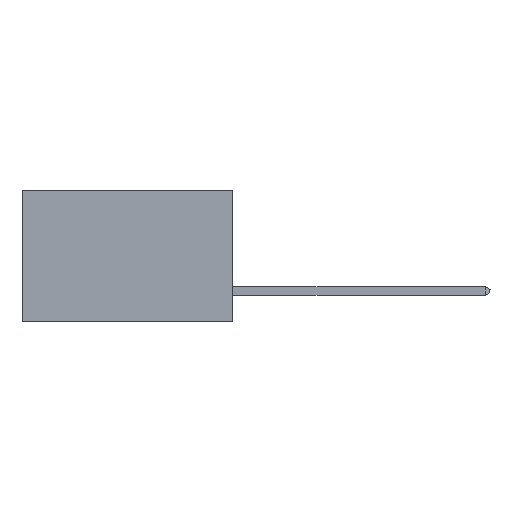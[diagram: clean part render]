
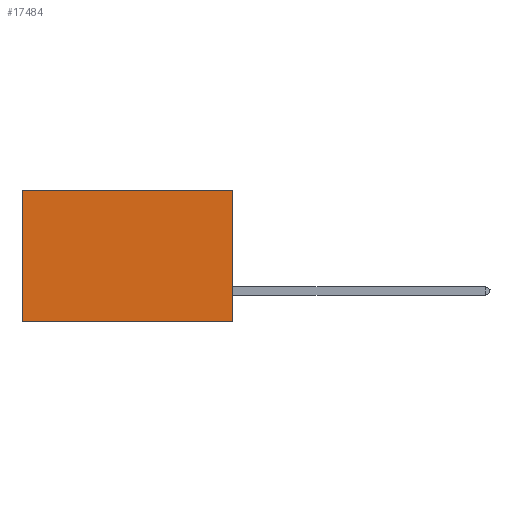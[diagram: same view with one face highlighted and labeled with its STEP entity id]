
A CAD part, left-side view. The second image highlights one B-rep face of the part: STEP entity #17484.
In plain terms, the highlighted planar face has unit normal (-1, 0, 0).
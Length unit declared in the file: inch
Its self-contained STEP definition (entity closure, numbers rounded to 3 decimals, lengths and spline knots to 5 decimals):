
#314 = VERTEX_POINT ( 'NONE', #1687 ) ;
#562 = VECTOR ( 'NONE', #758, 39.37008 ) ;
#758 = DIRECTION ( 'NONE',  ( 0., 0., -1. ) ) ;
#1687 = CARTESIAN_POINT ( 'NONE',  ( 0.2875, 0., -0.375 ) ) ;
#1917 = EDGE_LOOP ( 'NONE', ( #8400, #15700, #15957, #14129 ) ) ;
#2002 = VECTOR ( 'NONE', #3467, 39.37008 ) ;
#3012 = CARTESIAN_POINT ( 'NONE',  ( 0.2875, 0., -0.375 ) ) ;
#3467 = DIRECTION ( 'NONE',  ( 0., 1., 0. ) ) ;
#4912 = CARTESIAN_POINT ( 'NONE',  ( 0.2875, 0., 0. ) ) ;
#5191 = PLANE ( 'NONE',  #7289 ) ;
#7289 = AXIS2_PLACEMENT_3D ( 'NONE', #16228, #12255, #10941 ) ;
#7297 = EDGE_CURVE ( 'NONE', #16025, #314, #12103, .T. ) ;
#7659 = EDGE_CURVE ( 'NONE', #16231, #8420, #12306, .T. ) ;
#8114 = EDGE_CURVE ( 'NONE', #16025, #16231, #13351, .T. ) ;
#8400 = ORIENTED_EDGE ( 'NONE', *, *, #7659, .T. ) ;
#8420 = VERTEX_POINT ( 'NONE', #17685 ) ;
#8925 = FACE_OUTER_BOUND ( 'NONE', #1917, .T. ) ;
#9191 = CARTESIAN_POINT ( 'NONE',  ( 0.2875, 0.6, -0.375 ) ) ;
#10941 = DIRECTION ( 'NONE',  ( 0., 0., -1. ) ) ;
#11090 = VECTOR ( 'NONE', #11193, 39.37008 ) ;
#11193 = DIRECTION ( 'NONE',  ( 0., 1., 0. ) ) ;
#12103 = LINE ( 'NONE', #17065, #562 ) ;
#12255 = DIRECTION ( 'NONE',  ( 1., 0., 0. ) ) ;
#12306 = LINE ( 'NONE', #9191, #14635 ) ;
#13193 = DIRECTION ( 'NONE',  ( 0., 0., -1. ) ) ;
#13351 = LINE ( 'NONE', #4912, #2002 ) ;
#13662 = LINE ( 'NONE', #3012, #11090 ) ;
#14129 = ORIENTED_EDGE ( 'NONE', *, *, #8114, .T. ) ;
#14635 = VECTOR ( 'NONE', #13193, 39.37008 ) ;
#15700 = ORIENTED_EDGE ( 'NONE', *, *, #15866, .F. ) ;
#15866 = EDGE_CURVE ( 'NONE', #314, #8420, #13662, .T. ) ;
#15932 = CARTESIAN_POINT ( 'NONE',  ( 0.2875, 0.6, 0. ) ) ;
#15957 = ORIENTED_EDGE ( 'NONE', *, *, #7297, .F. ) ;
#16025 = VERTEX_POINT ( 'NONE', #17373 ) ;
#16228 = CARTESIAN_POINT ( 'NONE',  ( 0.2875, 0., -0.375 ) ) ;
#16231 = VERTEX_POINT ( 'NONE', #15932 ) ;
#17065 = CARTESIAN_POINT ( 'NONE',  ( 0.2875, 0., -0.375 ) ) ;
#17373 = CARTESIAN_POINT ( 'NONE',  ( 0.2875, 0., 0. ) ) ;
#17484 = ADVANCED_FACE ( 'NONE', ( #8925 ), #5191, .F. ) ;
#17685 = CARTESIAN_POINT ( 'NONE',  ( 0.2875, 0.6, -0.375 ) ) ;
